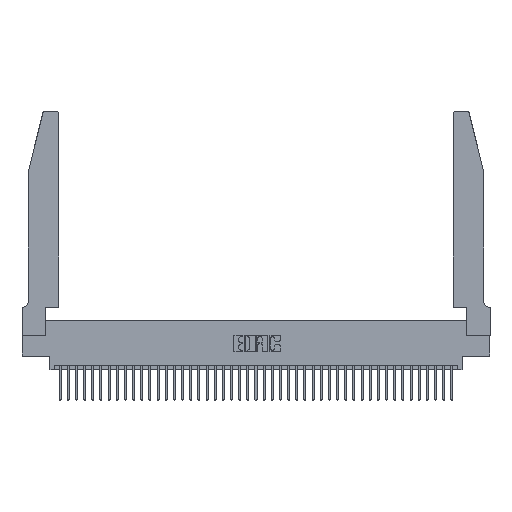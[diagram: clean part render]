
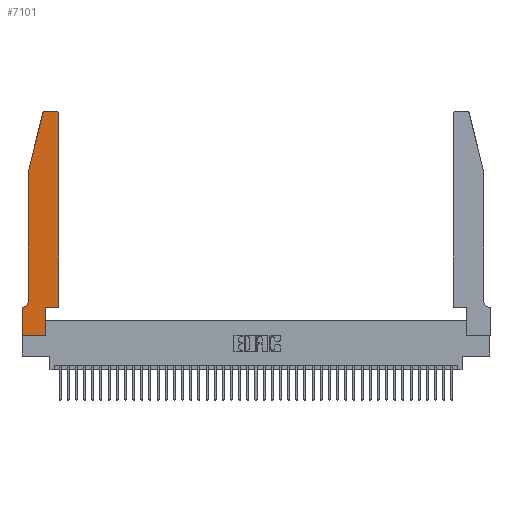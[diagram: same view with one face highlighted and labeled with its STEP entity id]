
A CAD part, top view. The second image highlights one B-rep face of the part: STEP entity #7101.
In plain terms, the highlighted planar face has unit normal (0, 0, 1).
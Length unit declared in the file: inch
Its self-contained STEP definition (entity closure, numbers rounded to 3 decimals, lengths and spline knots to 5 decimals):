
#15 = VERTEX_POINT ( 'NONE', #30454 ) ;
#408 = ORIENTED_EDGE ( 'NONE', *, *, #30525, .T. ) ;
#1031 = CARTESIAN_POINT ( 'NONE',  ( 0.2865, 0.35, 0.37 ) ) ;
#1644 = CARTESIAN_POINT ( 'NONE',  ( 0.4505, 2.72, 0.37 ) ) ;
#2725 = DIRECTION ( 'NONE',  ( -1., 0., 0. ) ) ;
#3021 = EDGE_CURVE ( 'NONE', #10366, #35957, #16571, .T. ) ;
#3464 = LINE ( 'NONE', #3739, #9141 ) ;
#3739 = CARTESIAN_POINT ( 'NONE',  ( 0.0755, 2., 0.37 ) ) ;
#3990 = LINE ( 'NONE', #35923, #39334 ) ;
#4141 = DIRECTION ( 'NONE',  ( 0., -1., 0. ) ) ;
#4454 = CARTESIAN_POINT ( 'NONE',  ( 0.4205, 2.75, 0.37 ) ) ;
#4973 = ORIENTED_EDGE ( 'NONE', *, *, #37668, .T. ) ;
#5147 = ORIENTED_EDGE ( 'NONE', *, *, #24970, .T. ) ;
#5162 = DIRECTION ( 'NONE',  ( 1., 0., 0. ) ) ;
#5239 = DIRECTION ( 'NONE',  ( 0., 0., 1. ) ) ;
#5536 = CARTESIAN_POINT ( 'NONE',  ( 0.2605, 2.75, 0.37 ) ) ;
#5622 = VERTEX_POINT ( 'NONE', #12785 ) ;
#5675 = VECTOR ( 'NONE', #26287, 39.37008 ) ;
#5773 = VERTEX_POINT ( 'NONE', #31984 ) ;
#6642 = DIRECTION ( 'NONE',  ( 1., 0., 0. ) ) ;
#7036 = VERTEX_POINT ( 'NONE', #20997 ) ;
#7101 = ADVANCED_FACE ( 'NONE', ( #26464 ), #37994, .T. ) ;
#7937 = ORIENTED_EDGE ( 'NONE', *, *, #3021, .T. ) ;
#8055 = DIRECTION ( 'NONE',  ( 0., 0., 1. ) ) ;
#8242 = VECTOR ( 'NONE', #24985, 39.37008 ) ;
#9141 = VECTOR ( 'NONE', #38706, 39.37008 ) ;
#9807 = CIRCLE ( 'NONE', #40225, 0.03 ) ;
#10093 = VERTEX_POINT ( 'NONE', #34955 ) ;
#10366 = VERTEX_POINT ( 'NONE', #1644 ) ;
#10813 = EDGE_CURVE ( 'NONE', #5622, #20593, #37399, .T. ) ;
#11538 = CARTESIAN_POINT ( 'NONE',  ( 0., 0.35, 0.37 ) ) ;
#11760 = VERTEX_POINT ( 'NONE', #38515 ) ;
#11933 = CARTESIAN_POINT ( 'NONE',  ( 0.284, 2.75, 0.37 ) ) ;
#12265 = EDGE_CURVE ( 'NONE', #15832, #15, #33745, .T. ) ;
#12577 = EDGE_CURVE ( 'NONE', #15, #10366, #21924, .T. ) ;
#12785 = CARTESIAN_POINT ( 'NONE',  ( 0.25487, 2.72718, 0.37 ) ) ;
#13197 = VECTOR ( 'NONE', #24177, 39.37008 ) ;
#13542 = EDGE_CURVE ( 'NONE', #7036, #10093, #3990, .T. ) ;
#13888 = AXIS2_PLACEMENT_3D ( 'NONE', #17351, #20091, #39842 ) ;
#14305 = EDGE_LOOP ( 'NONE', ( #26930, #408, #25905, #5147, #26480, #39905, #30147, #37764, #4973, #24378, #18223, #7937 ) ) ;
#14682 = LINE ( 'NONE', #1031, #15691 ) ;
#15691 = VECTOR ( 'NONE', #30340, 39.37008 ) ;
#15832 = VERTEX_POINT ( 'NONE', #37258 ) ;
#16571 = CIRCLE ( 'NONE', #32924, 0.03 ) ;
#17351 = CARTESIAN_POINT ( 'NONE',  ( 0.0055, 0.42, 0.37 ) ) ;
#18181 = DIRECTION ( 'NONE',  ( 1., 0., 0. ) ) ;
#18223 = ORIENTED_EDGE ( 'NONE', *, *, #12577, .T. ) ;
#18310 = VECTOR ( 'NONE', #5162, 39.37008 ) ;
#18473 = LINE ( 'NONE', #38122, #8242 ) ;
#18597 = EDGE_CURVE ( 'NONE', #35957, #25075, #20479, .T. ) ;
#18621 = EDGE_CURVE ( 'NONE', #11760, #7036, #30282, .T. ) ;
#20091 = DIRECTION ( 'NONE',  ( 0., 0., -1. ) ) ;
#20479 = LINE ( 'NONE', #5536, #5675 ) ;
#20593 = VERTEX_POINT ( 'NONE', #22862 ) ;
#20885 = CARTESIAN_POINT ( 'NONE',  ( 0., 0., 0.37 ) ) ;
#20997 = CARTESIAN_POINT ( 'NONE',  ( 0.0055, 0.35, 0.37 ) ) ;
#21924 = LINE ( 'NONE', #24035, #13197 ) ;
#21931 = LINE ( 'NONE', #20885, #25002 ) ;
#22862 = CARTESIAN_POINT ( 'NONE',  ( 0.0755, 2., 0.37 ) ) ;
#22952 = DIRECTION ( 'NONE',  ( 0., 0., 1. ) ) ;
#24035 = CARTESIAN_POINT ( 'NONE',  ( 0.4505, 0.35, 0.37 ) ) ;
#24177 = DIRECTION ( 'NONE',  ( 0., 1., 0. ) ) ;
#24378 = ORIENTED_EDGE ( 'NONE', *, *, #12265, .T. ) ;
#24970 = EDGE_CURVE ( 'NONE', #20593, #11760, #3464, .T. ) ;
#24985 = DIRECTION ( 'NONE',  ( 1., 0., 0. ) ) ;
#25002 = VECTOR ( 'NONE', #4141, 39.37008 ) ;
#25075 = VERTEX_POINT ( 'NONE', #11933 ) ;
#25905 = ORIENTED_EDGE ( 'NONE', *, *, #10813, .T. ) ;
#26121 = CARTESIAN_POINT ( 'NONE',  ( 0.4205, 2.72, 0.37 ) ) ;
#26287 = DIRECTION ( 'NONE',  ( -1., 0., 0. ) ) ;
#26464 = FACE_OUTER_BOUND ( 'NONE', #14305, .T. ) ;
#26480 = ORIENTED_EDGE ( 'NONE', *, *, #18621, .T. ) ;
#26930 = ORIENTED_EDGE ( 'NONE', *, *, #18597, .T. ) ;
#29817 = DIRECTION ( 'NONE',  ( -0.239, -0.971, 0. ) ) ;
#30147 = ORIENTED_EDGE ( 'NONE', *, *, #41350, .T. ) ;
#30282 = CIRCLE ( 'NONE', #13888, 0.07 ) ;
#30340 = DIRECTION ( 'NONE',  ( 0., 1., 0. ) ) ;
#30377 = CARTESIAN_POINT ( 'NONE',  ( 0.2865, 0., 0.37 ) ) ;
#30454 = CARTESIAN_POINT ( 'NONE',  ( 0.4505, 0.35, 0.37 ) ) ;
#30525 = EDGE_CURVE ( 'NONE', #25075, #5622, #9807, .T. ) ;
#31984 = CARTESIAN_POINT ( 'NONE',  ( 0., 0., 0.37 ) ) ;
#32495 = AXIS2_PLACEMENT_3D ( 'NONE', #11538, #5239, #34448 ) ;
#32924 = AXIS2_PLACEMENT_3D ( 'NONE', #26121, #22952, #6642 ) ;
#33745 = LINE ( 'NONE', #37915, #18310 ) ;
#34448 = DIRECTION ( 'NONE',  ( 1., 0., 0. ) ) ;
#34955 = CARTESIAN_POINT ( 'NONE',  ( 0., 0.35, 0.37 ) ) ;
#35297 = EDGE_CURVE ( 'NONE', #5773, #39278, #18473, .T. ) ;
#35923 = CARTESIAN_POINT ( 'NONE',  ( 0.0755, 0.35, 0.37 ) ) ;
#35957 = VERTEX_POINT ( 'NONE', #4454 ) ;
#37202 = CARTESIAN_POINT ( 'NONE',  ( 0.0755, 2., 0.37 ) ) ;
#37258 = CARTESIAN_POINT ( 'NONE',  ( 0.2865, 0.35, 0.37 ) ) ;
#37399 = LINE ( 'NONE', #37202, #40506 ) ;
#37668 = EDGE_CURVE ( 'NONE', #39278, #15832, #14682, .T. ) ;
#37764 = ORIENTED_EDGE ( 'NONE', *, *, #35297, .T. ) ;
#37811 = CARTESIAN_POINT ( 'NONE',  ( 0.284, 2.72, 0.37 ) ) ;
#37915 = CARTESIAN_POINT ( 'NONE',  ( 0.4505, 0.35, 0.37 ) ) ;
#37994 = PLANE ( 'NONE',  #32495 ) ;
#38122 = CARTESIAN_POINT ( 'NONE',  ( 0., 0., 0.37 ) ) ;
#38515 = CARTESIAN_POINT ( 'NONE',  ( 0.0755, 0.42, 0.37 ) ) ;
#38706 = DIRECTION ( 'NONE',  ( 0., -1., 0. ) ) ;
#39278 = VERTEX_POINT ( 'NONE', #30377 ) ;
#39334 = VECTOR ( 'NONE', #2725, 39.37008 ) ;
#39842 = DIRECTION ( 'NONE',  ( -1., 0., 0. ) ) ;
#39905 = ORIENTED_EDGE ( 'NONE', *, *, #13542, .T. ) ;
#40225 = AXIS2_PLACEMENT_3D ( 'NONE', #37811, #8055, #18181 ) ;
#40506 = VECTOR ( 'NONE', #29817, 39.37008 ) ;
#41350 = EDGE_CURVE ( 'NONE', #10093, #5773, #21931, .T. ) ;
